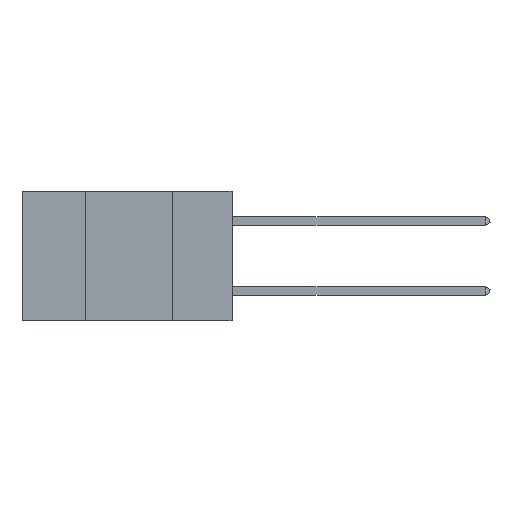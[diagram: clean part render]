
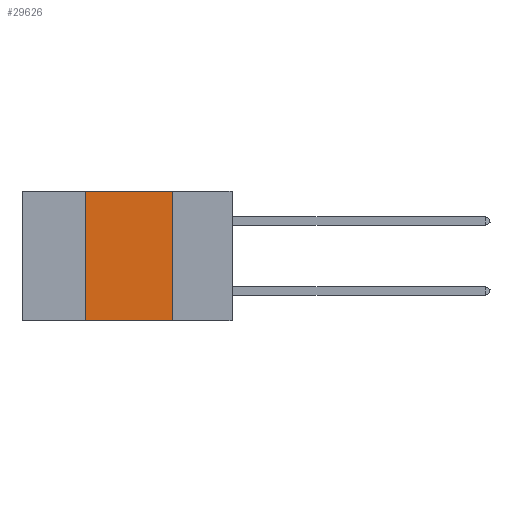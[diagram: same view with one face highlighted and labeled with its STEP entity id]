
A CAD part, left-side view. The second image highlights one B-rep face of the part: STEP entity #29626.
In plain terms, the highlighted planar face has unit normal (-1, 0, 0).
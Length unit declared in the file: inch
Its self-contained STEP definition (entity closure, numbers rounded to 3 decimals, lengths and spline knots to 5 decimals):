
#245 = CARTESIAN_POINT ( 'NONE',  ( 0., 0.17, 0. ) ) ;
#2431 = ORIENTED_EDGE ( 'NONE', *, *, #19802, .F. ) ;
#2916 = VERTEX_POINT ( 'NONE', #3759 ) ;
#3354 = CARTESIAN_POINT ( 'NONE',  ( 0., 0.6, 0. ) ) ;
#3759 = CARTESIAN_POINT ( 'NONE',  ( 0., 0.17, 0. ) ) ;
#4635 = CARTESIAN_POINT ( 'NONE',  ( 0., 0.42, 0. ) ) ;
#5994 = EDGE_CURVE ( 'NONE', #2916, #31718, #16936, .T. ) ;
#6670 = VECTOR ( 'NONE', #26707, 39.37008 ) ;
#7838 = DIRECTION ( 'NONE',  ( 0., 0., 1. ) ) ;
#8475 = CARTESIAN_POINT ( 'NONE',  ( 0., 0.6, -0.37 ) ) ;
#9684 = VECTOR ( 'NONE', #25887, 39.37008 ) ;
#10749 = PLANE ( 'NONE',  #12317 ) ;
#11369 = CARTESIAN_POINT ( 'NONE',  ( 0., 0.42, -0.37 ) ) ;
#12317 = AXIS2_PLACEMENT_3D ( 'NONE', #3354, #18304, #21328 ) ;
#13358 = LINE ( 'NONE', #23633, #32976 ) ;
#14958 = EDGE_LOOP ( 'NONE', ( #22459, #2431, #31751, #17591 ) ) ;
#15991 = CARTESIAN_POINT ( 'NONE',  ( 0., 0.6, 0. ) ) ;
#16072 = VERTEX_POINT ( 'NONE', #4635 ) ;
#16936 = LINE ( 'NONE', #245, #9684 ) ;
#17016 = EDGE_CURVE ( 'NONE', #28269, #31718, #24615, .T. ) ;
#17591 = ORIENTED_EDGE ( 'NONE', *, *, #17016, .T. ) ;
#18304 = DIRECTION ( 'NONE',  ( 1., 0., 0. ) ) ;
#18345 = EDGE_CURVE ( 'NONE', #28269, #16072, #13358, .T. ) ;
#19537 = LINE ( 'NONE', #15991, #6670 ) ;
#19802 = EDGE_CURVE ( 'NONE', #16072, #2916, #19537, .T. ) ;
#21328 = DIRECTION ( 'NONE',  ( 0., 0., -1. ) ) ;
#22459 = ORIENTED_EDGE ( 'NONE', *, *, #5994, .F. ) ;
#23633 = CARTESIAN_POINT ( 'NONE',  ( 0., 0.42, 0. ) ) ;
#24615 = LINE ( 'NONE', #8475, #30213 ) ;
#25887 = DIRECTION ( 'NONE',  ( 0., 0., -1. ) ) ;
#26294 = FACE_OUTER_BOUND ( 'NONE', #14958, .T. ) ;
#26707 = DIRECTION ( 'NONE',  ( 0., -1., 0. ) ) ;
#28269 = VERTEX_POINT ( 'NONE', #11369 ) ;
#29626 = ADVANCED_FACE ( 'NONE', ( #26294 ), #10749, .F. ) ;
#30213 = VECTOR ( 'NONE', #31512, 39.37008 ) ;
#31512 = DIRECTION ( 'NONE',  ( 0., -1., 0. ) ) ;
#31718 = VERTEX_POINT ( 'NONE', #31731 ) ;
#31731 = CARTESIAN_POINT ( 'NONE',  ( 0., 0.17, -0.37 ) ) ;
#31751 = ORIENTED_EDGE ( 'NONE', *, *, #18345, .F. ) ;
#32976 = VECTOR ( 'NONE', #7838, 39.37008 ) ;
